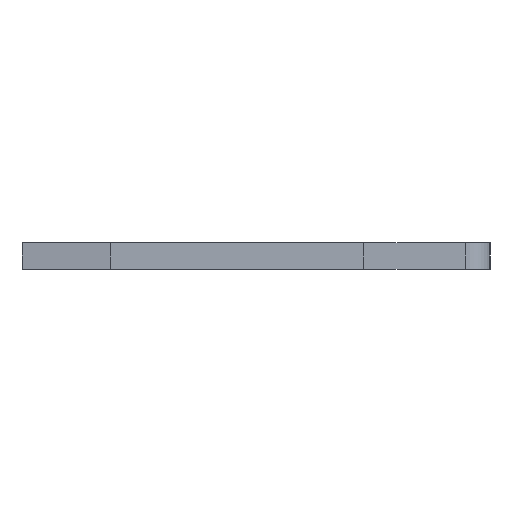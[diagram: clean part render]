
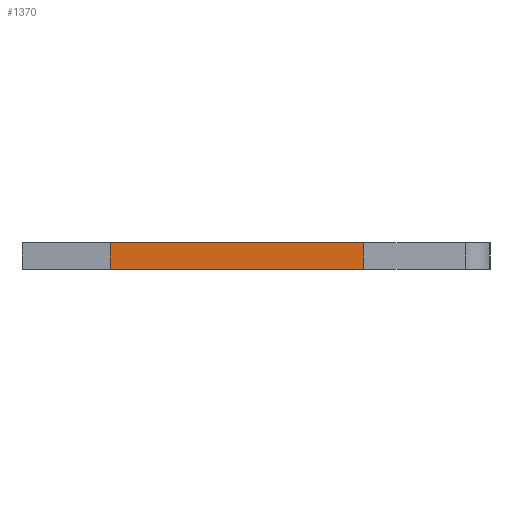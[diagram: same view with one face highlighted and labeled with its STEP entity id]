
A CAD part, left-side view. The second image highlights one B-rep face of the part: STEP entity #1370.
In plain terms, the highlighted face is planar.
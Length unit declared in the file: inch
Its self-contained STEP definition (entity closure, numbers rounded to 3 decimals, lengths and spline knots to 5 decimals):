
#17 = VECTOR ( 'NONE', #802, 39.37008 ) ;
#41 = ORIENTED_EDGE ( 'NONE', *, *, #211, .F. ) ;
#50 = VERTEX_POINT ( 'NONE', #624 ) ;
#91 = VECTOR ( 'NONE', #715, 39.37008 ) ;
#211 = EDGE_CURVE ( 'NONE', #50, #1538, #1516, .T. ) ;
#275 = VECTOR ( 'NONE', #618, 39.37008 ) ;
#302 = LINE ( 'NONE', #1354, #275 ) ;
#313 = DIRECTION ( 'NONE',  ( 0., 0., 1. ) ) ;
#409 = DIRECTION ( 'NONE',  ( 1., 0., 0. ) ) ;
#416 = CARTESIAN_POINT ( 'NONE',  ( 0.013, 0.146, -0.0575 ) ) ;
#422 = VERTEX_POINT ( 'NONE', #1047 ) ;
#440 = LINE ( 'NONE', #460, #91 ) ;
#460 = CARTESIAN_POINT ( 'NONE',  ( 0.013, -0.099, -0.0575 ) ) ;
#535 = CARTESIAN_POINT ( 'NONE',  ( 0.013, 0.146, -0.0575 ) ) ;
#615 = ORIENTED_EDGE ( 'NONE', *, *, #776, .T. ) ;
#618 = DIRECTION ( 'NONE',  ( 0., 1., 0. ) ) ;
#624 = CARTESIAN_POINT ( 'NONE',  ( 0.013, -0.099, -0.0575 ) ) ;
#639 = CARTESIAN_POINT ( 'NONE',  ( 0.013, 0.146, -0.0575 ) ) ;
#658 = EDGE_LOOP ( 'NONE', ( #1270, #1043, #41, #615 ) ) ;
#715 = DIRECTION ( 'NONE',  ( -1., 0., 0. ) ) ;
#776 = EDGE_CURVE ( 'NONE', #50, #422, #440, .T. ) ;
#792 = PLANE ( 'NONE',  #1033 ) ;
#796 = CARTESIAN_POINT ( 'NONE',  ( 0.013, 0.146, -0.0575 ) ) ;
#802 = DIRECTION ( 'NONE',  ( 0., 1., 0. ) ) ;
#908 = VERTEX_POINT ( 'NONE', #1358 ) ;
#1020 = DIRECTION ( 'NONE',  ( -1., 0., 0. ) ) ;
#1033 = AXIS2_PLACEMENT_3D ( 'NONE', #535, #313, #409 ) ;
#1043 = ORIENTED_EDGE ( 'NONE', *, *, #1268, .F. ) ;
#1047 = CARTESIAN_POINT ( 'NONE',  ( -0.013, -0.099, -0.0575 ) ) ;
#1095 = EDGE_CURVE ( 'NONE', #422, #908, #302, .T. ) ;
#1132 = VECTOR ( 'NONE', #1020, 39.37008 ) ;
#1213 = LINE ( 'NONE', #639, #1132 ) ;
#1268 = EDGE_CURVE ( 'NONE', #1538, #908, #1213, .T. ) ;
#1270 = ORIENTED_EDGE ( 'NONE', *, *, #1095, .T. ) ;
#1354 = CARTESIAN_POINT ( 'NONE',  ( -0.013, 0.146, -0.0575 ) ) ;
#1358 = CARTESIAN_POINT ( 'NONE',  ( -0.013, 0.146, -0.0575 ) ) ;
#1370 = ADVANCED_FACE ( 'NONE', ( #1406 ), #792, .F. ) ;
#1406 = FACE_OUTER_BOUND ( 'NONE', #658, .T. ) ;
#1516 = LINE ( 'NONE', #796, #17 ) ;
#1538 = VERTEX_POINT ( 'NONE', #416 ) ;
